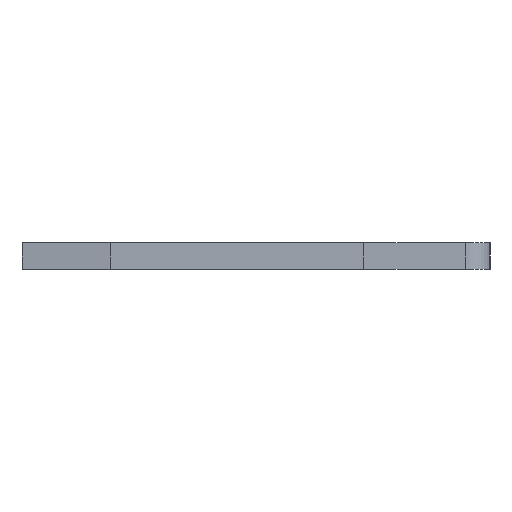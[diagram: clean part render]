
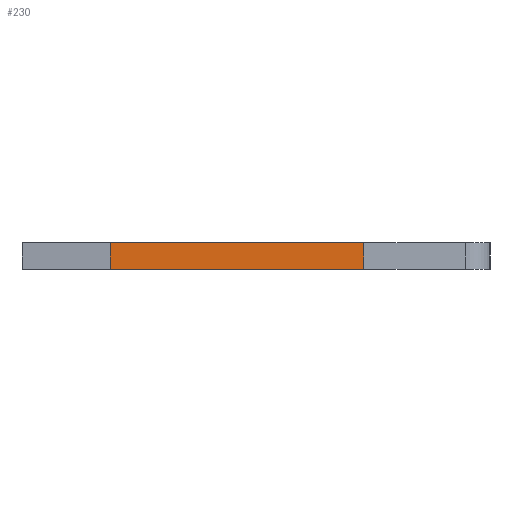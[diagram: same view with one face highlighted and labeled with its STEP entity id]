
A CAD part, left-side view. The second image highlights one B-rep face of the part: STEP entity #230.
In plain terms, the highlighted face is planar.
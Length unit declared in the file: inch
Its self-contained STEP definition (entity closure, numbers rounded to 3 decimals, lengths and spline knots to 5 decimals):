
#138 = EDGE_LOOP ( 'NONE', ( #726, #319, #445, #587 ) ) ;
#177 = DIRECTION ( 'NONE',  ( 0., 1., 0. ) ) ;
#230 = ADVANCED_FACE ( 'NONE', ( #1022 ), #975, .F. ) ;
#311 = VECTOR ( 'NONE', #631, 39.37008 ) ;
#319 = ORIENTED_EDGE ( 'NONE', *, *, #1055, .F. ) ;
#382 = VECTOR ( 'NONE', #1241, 39.37008 ) ;
#390 = CARTESIAN_POINT ( 'NONE',  ( -0.013, 0.146, -0.0575 ) ) ;
#395 = CARTESIAN_POINT ( 'NONE',  ( -0.013, 0.146, -0.0575 ) ) ;
#445 = ORIENTED_EDGE ( 'NONE', *, *, #894, .F. ) ;
#484 = VECTOR ( 'NONE', #609, 39.37008 ) ;
#502 = CARTESIAN_POINT ( 'NONE',  ( 0.013, -0.099, -0.0575 ) ) ;
#556 = AXIS2_PLACEMENT_3D ( 'NONE', #1061, #1073, #969 ) ;
#559 = VERTEX_POINT ( 'NONE', #781 ) ;
#587 = ORIENTED_EDGE ( 'NONE', *, *, #893, .T. ) ;
#609 = DIRECTION ( 'NONE',  ( 0., 1., 0. ) ) ;
#612 = CARTESIAN_POINT ( 'NONE',  ( 0.013, 0.146, -0.0575 ) ) ;
#631 = DIRECTION ( 'NONE',  ( -1., 0., 0. ) ) ;
#634 = VERTEX_POINT ( 'NONE', #1125 ) ;
#726 = ORIENTED_EDGE ( 'NONE', *, *, #859, .T. ) ;
#781 = CARTESIAN_POINT ( 'NONE',  ( 0.013, -0.099, -0.0575 ) ) ;
#846 = LINE ( 'NONE', #502, #382 ) ;
#859 = EDGE_CURVE ( 'NONE', #634, #971, #1018, .T. ) ;
#863 = VERTEX_POINT ( 'NONE', #1031 ) ;
#865 = LINE ( 'NONE', #612, #484 ) ;
#893 = EDGE_CURVE ( 'NONE', #559, #634, #846, .T. ) ;
#894 = EDGE_CURVE ( 'NONE', #559, #863, #865, .T. ) ;
#903 = VECTOR ( 'NONE', #177, 39.37008 ) ;
#969 = DIRECTION ( 'NONE',  ( 1., 0., 0. ) ) ;
#971 = VERTEX_POINT ( 'NONE', #390 ) ;
#975 = PLANE ( 'NONE',  #556 ) ;
#1018 = LINE ( 'NONE', #395, #903 ) ;
#1022 = FACE_OUTER_BOUND ( 'NONE', #138, .T. ) ;
#1031 = CARTESIAN_POINT ( 'NONE',  ( 0.013, 0.146, -0.0575 ) ) ;
#1052 = CARTESIAN_POINT ( 'NONE',  ( 0.013, 0.146, -0.0575 ) ) ;
#1055 = EDGE_CURVE ( 'NONE', #863, #971, #1231, .T. ) ;
#1061 = CARTESIAN_POINT ( 'NONE',  ( 0.013, 0.146, -0.0575 ) ) ;
#1073 = DIRECTION ( 'NONE',  ( 0., 0., 1. ) ) ;
#1125 = CARTESIAN_POINT ( 'NONE',  ( -0.013, -0.099, -0.0575 ) ) ;
#1231 = LINE ( 'NONE', #1052, #311 ) ;
#1241 = DIRECTION ( 'NONE',  ( -1., 0., 0. ) ) ;
